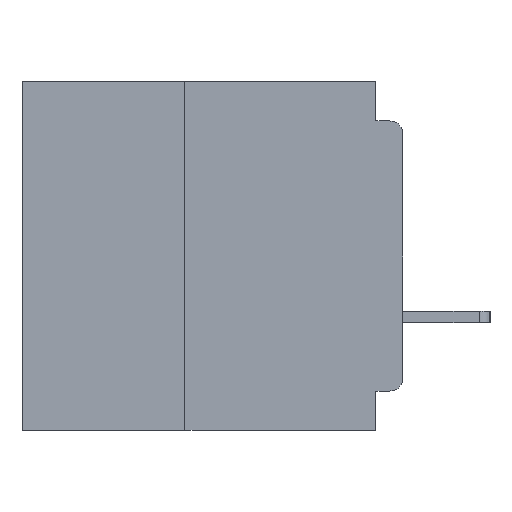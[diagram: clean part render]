
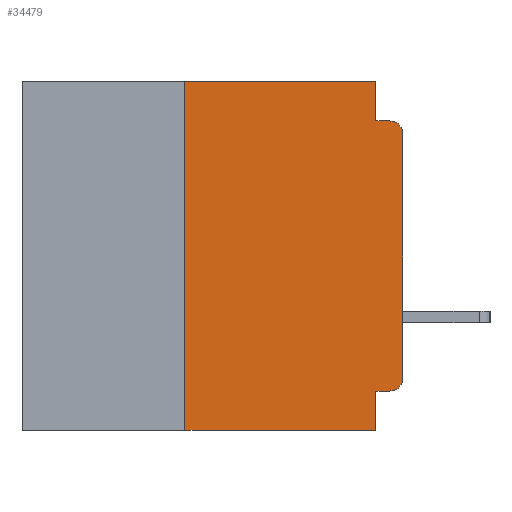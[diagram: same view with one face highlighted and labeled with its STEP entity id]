
A CAD part, left-side view. The second image highlights one B-rep face of the part: STEP entity #34479.
In plain terms, the highlighted planar face has unit normal (-1, 0, 0).
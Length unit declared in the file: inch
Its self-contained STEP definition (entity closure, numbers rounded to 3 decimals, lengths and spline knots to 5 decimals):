
#295 = FACE_OUTER_BOUND ( 'NONE', #20542, .T. ) ;
#1211 = CARTESIAN_POINT ( 'NONE',  ( 0., 0.437, 0. ) ) ;
#1229 = EDGE_CURVE ( 'NONE', #15876, #20025, #19052, .T. ) ;
#2856 = LINE ( 'NONE', #4263, #36920 ) ;
#3394 = LINE ( 'NONE', #24684, #12284 ) ;
#3395 = VECTOR ( 'NONE', #40389, 39.37008 ) ;
#4239 = EDGE_CURVE ( 'NONE', #16254, #16773, #5787, .T. ) ;
#4263 = CARTESIAN_POINT ( 'NONE',  ( 0., 0.031, 0. ) ) ;
#4412 = CIRCLE ( 'NONE', #38645, 0.015 ) ;
#4591 = DIRECTION ( 'NONE',  ( 0., 0., -1. ) ) ;
#4771 = DIRECTION ( 'NONE',  ( 0., -1., 0. ) ) ;
#5105 = CARTESIAN_POINT ( 'NONE',  ( 0., 0., -0.355 ) ) ;
#5651 = VECTOR ( 'NONE', #31428, 39.37008 ) ;
#5787 = LINE ( 'NONE', #13851, #13661 ) ;
#6108 = DIRECTION ( 'NONE',  ( 0., 0., 1. ) ) ;
#6463 = VECTOR ( 'NONE', #35144, 39.37008 ) ;
#7448 = ORIENTED_EDGE ( 'NONE', *, *, #1229, .T. ) ;
#8262 = CARTESIAN_POINT ( 'NONE',  ( 0., 0.015, -0.34 ) ) ;
#8778 = CARTESIAN_POINT ( 'NONE',  ( 0., 0.015, -0.06 ) ) ;
#8796 = CARTESIAN_POINT ( 'NONE',  ( 0., 0., -0.34 ) ) ;
#11134 = ORIENTED_EDGE ( 'NONE', *, *, #15722, .F. ) ;
#11136 = VERTEX_POINT ( 'NONE', #40936 ) ;
#11622 = DIRECTION ( 'NONE',  ( 0., 0., -1. ) ) ;
#12072 = ORIENTED_EDGE ( 'NONE', *, *, #22463, .F. ) ;
#12140 = DIRECTION ( 'NONE',  ( 0., 0., -1. ) ) ;
#12284 = VECTOR ( 'NONE', #4771, 39.37008 ) ;
#13661 = VECTOR ( 'NONE', #30206, 39.37008 ) ;
#13851 = CARTESIAN_POINT ( 'NONE',  ( 0., 0., 0. ) ) ;
#14013 = AXIS2_PLACEMENT_3D ( 'NONE', #8262, #31314, #11622 ) ;
#14818 = ORIENTED_EDGE ( 'NONE', *, *, #27105, .F. ) ;
#15312 = LINE ( 'NONE', #5105, #40293 ) ;
#15610 = ORIENTED_EDGE ( 'NONE', *, *, #29466, .F. ) ;
#15722 = EDGE_CURVE ( 'NONE', #23240, #40314, #32792, .T. ) ;
#15876 = VERTEX_POINT ( 'NONE', #17012 ) ;
#16254 = VERTEX_POINT ( 'NONE', #8796 ) ;
#16773 = VERTEX_POINT ( 'NONE', #30683 ) ;
#17012 = CARTESIAN_POINT ( 'NONE',  ( 0., 0.25, -0.4 ) ) ;
#17504 = EDGE_CURVE ( 'NONE', #36105, #16254, #21934, .T. ) ;
#18011 = EDGE_CURVE ( 'NONE', #40314, #11136, #2856, .T. ) ;
#18201 = EDGE_CURVE ( 'NONE', #16773, #38546, #4412, .T. ) ;
#19052 = LINE ( 'NONE', #40338, #3395 ) ;
#20025 = VERTEX_POINT ( 'NONE', #27823 ) ;
#20542 = EDGE_LOOP ( 'NONE', ( #22056, #24783, #34817, #41962, #11134, #12072, #7448, #15610, #14818, #27801 ) ) ;
#21934 = CIRCLE ( 'NONE', #14013, 0.015 ) ;
#22056 = ORIENTED_EDGE ( 'NONE', *, *, #4239, .T. ) ;
#22291 = LINE ( 'NONE', #29284, #29955 ) ;
#22463 = EDGE_CURVE ( 'NONE', #15876, #23240, #22291, .T. ) ;
#23240 = VERTEX_POINT ( 'NONE', #33164 ) ;
#24038 = VERTEX_POINT ( 'NONE', #37381 ) ;
#24386 = LINE ( 'NONE', #24926, #5651 ) ;
#24516 = DIRECTION ( 'NONE',  ( 1., 0., 0. ) ) ;
#24684 = CARTESIAN_POINT ( 'NONE',  ( 0., 0., -0.045 ) ) ;
#24783 = ORIENTED_EDGE ( 'NONE', *, *, #18201, .T. ) ;
#24926 = CARTESIAN_POINT ( 'NONE',  ( 0., 0.031, -0.4 ) ) ;
#25855 = EDGE_CURVE ( 'NONE', #11136, #38546, #3394, .T. ) ;
#27105 = EDGE_CURVE ( 'NONE', #36105, #24038, #15312, .T. ) ;
#27801 = ORIENTED_EDGE ( 'NONE', *, *, #17504, .T. ) ;
#27823 = CARTESIAN_POINT ( 'NONE',  ( 0., 0.031, -0.4 ) ) ;
#28087 = AXIS2_PLACEMENT_3D ( 'NONE', #1211, #24516, #4591 ) ;
#28287 = DIRECTION ( 'NONE',  ( 0., 1., 0. ) ) ;
#28627 = CARTESIAN_POINT ( 'NONE',  ( 0., 0.437, 0. ) ) ;
#29284 = CARTESIAN_POINT ( 'NONE',  ( 0., 0.25, -0.4 ) ) ;
#29466 = EDGE_CURVE ( 'NONE', #24038, #20025, #24386, .T. ) ;
#29934 = CARTESIAN_POINT ( 'NONE',  ( 0., 0.015, -0.355 ) ) ;
#29955 = VECTOR ( 'NONE', #6108, 39.37008 ) ;
#30206 = DIRECTION ( 'NONE',  ( 0., 0., 1. ) ) ;
#30683 = CARTESIAN_POINT ( 'NONE',  ( 0., 0., -0.06 ) ) ;
#31314 = DIRECTION ( 'NONE',  ( -1., 0., 0. ) ) ;
#31428 = DIRECTION ( 'NONE',  ( 0., 0., -1. ) ) ;
#31816 = DIRECTION ( 'NONE',  ( -1., 0., 0. ) ) ;
#32792 = LINE ( 'NONE', #28627, #6463 ) ;
#33164 = CARTESIAN_POINT ( 'NONE',  ( 0., 0.25, 0. ) ) ;
#34157 = PLANE ( 'NONE',  #28087 ) ;
#34479 = ADVANCED_FACE ( 'NONE', ( #295 ), #34157, .F. ) ;
#34817 = ORIENTED_EDGE ( 'NONE', *, *, #25855, .F. ) ;
#35144 = DIRECTION ( 'NONE',  ( 0., -1., 0. ) ) ;
#36105 = VERTEX_POINT ( 'NONE', #29934 ) ;
#36920 = VECTOR ( 'NONE', #37260, 39.37008 ) ;
#37260 = DIRECTION ( 'NONE',  ( 0., 0., -1. ) ) ;
#37381 = CARTESIAN_POINT ( 'NONE',  ( 0., 0.031, -0.355 ) ) ;
#37550 = CARTESIAN_POINT ( 'NONE',  ( 0., 0.015, -0.045 ) ) ;
#38546 = VERTEX_POINT ( 'NONE', #37550 ) ;
#38645 = AXIS2_PLACEMENT_3D ( 'NONE', #8778, #31816, #12140 ) ;
#39111 = CARTESIAN_POINT ( 'NONE',  ( 0., 0.031, 0. ) ) ;
#40293 = VECTOR ( 'NONE', #28287, 39.37008 ) ;
#40314 = VERTEX_POINT ( 'NONE', #39111 ) ;
#40338 = CARTESIAN_POINT ( 'NONE',  ( 0., 0.437, -0.4 ) ) ;
#40389 = DIRECTION ( 'NONE',  ( 0., -1., 0. ) ) ;
#40936 = CARTESIAN_POINT ( 'NONE',  ( 0., 0.031, -0.045 ) ) ;
#41962 = ORIENTED_EDGE ( 'NONE', *, *, #18011, .F. ) ;
